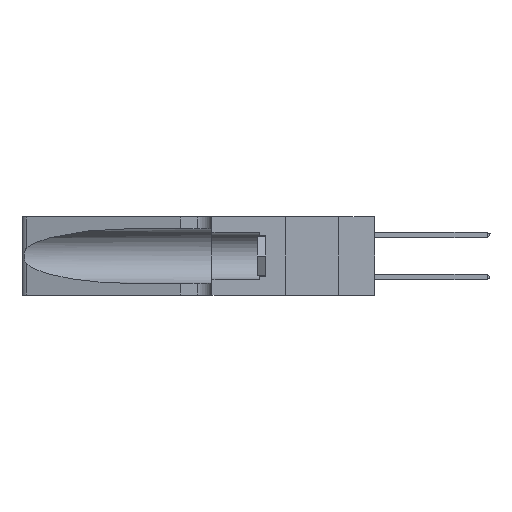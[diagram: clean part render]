
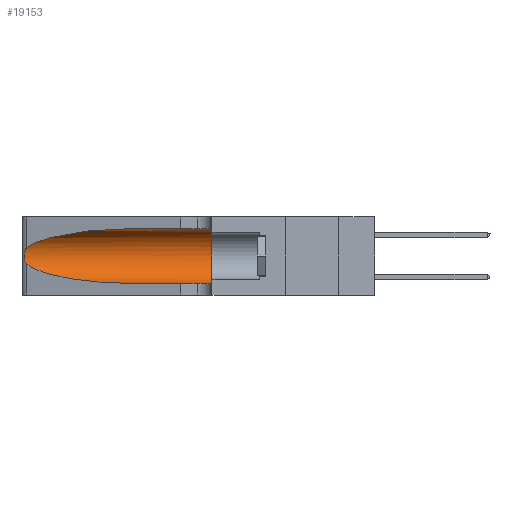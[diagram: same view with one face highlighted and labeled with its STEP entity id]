
A CAD part, left-side view. The second image highlights one B-rep face of the part: STEP entity #19153.
In plain terms, the highlighted cylindrical face has radius 3.308 mm (diameter 6.617 mm), a partial arc.
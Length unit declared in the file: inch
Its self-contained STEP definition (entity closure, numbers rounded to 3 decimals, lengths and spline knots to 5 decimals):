
#128 = EDGE_LOOP ( 'NONE', ( #16475, #12457, #3145, #19576, #9254, #17117 ) ) ;
#361 = CARTESIAN_POINT ( 'NONE',  ( 0.1305, 1.61858, 0.31525 ) ) ;
#1001 = CARTESIAN_POINT ( 'NONE',  ( 0.1305, 0.72297, 0.31525 ) ) ;
#1031 = DIRECTION ( 'NONE',  ( 0., -1., 0. ) ) ;
#1089 = CARTESIAN_POINT ( 'NONE',  ( 0.2373, 1.15595, 0.28018 ) ) ;
#1699 = AXIS2_PLACEMENT_3D ( 'NONE', #20190, #12353, #16362 ) ;
#2793 = VERTEX_POINT ( 'NONE', #5870 ) ;
#2833 = VERTEX_POINT ( 'NONE', #12127 ) ;
#3140 = EDGE_CURVE ( 'NONE', #2793, #24458, #7477, .T. ) ;
#3145 = ORIENTED_EDGE ( 'NONE', *, *, #16802, .T. ) ;
#3312 =( BOUNDED_CURVE ( )  B_SPLINE_CURVE ( 3, ( #18362, #6583, #24259, #16506 ),
 .UNSPECIFIED., .F., .F. ) 
 B_SPLINE_CURVE_WITH_KNOTS ( ( 4, 4 ),
 ( 3.44316, 4.71239 ),
 .UNSPECIFIED. ) 
 CURVE ( )  GEOMETRIC_REPRESENTATION_ITEM ( )  RATIONAL_B_SPLINE_CURVE ( ( 1., 0.87, 0.87, 1. ) ) 
 REPRESENTATION_ITEM ( '' )  );
#3843 = CARTESIAN_POINT ( 'NONE',  ( 0.25787, 1.23484, 0.2124 ) ) ;
#4177 = CARTESIAN_POINT ( 'NONE',  ( 0.25856, 1.23593, 0.16098 ) ) ;
#4266 = VERTEX_POINT ( 'NONE', #18389 ) ;
#4960 = CARTESIAN_POINT ( 'NONE',  ( 0.18966, 0.96281, 0.31525 ) ) ;
#5870 = CARTESIAN_POINT ( 'NONE',  ( 0.1305, 0.72297, 0.31525 ) ) ;
#6583 = CARTESIAN_POINT ( 'NONE',  ( 0.2373, 1.15595, 0.08982 ) ) ;
#6939 = CARTESIAN_POINT ( 'NONE',  ( 0.1305, 0.35, 0.05475 ) ) ;
#7477 =( BOUNDED_CURVE ( )  B_SPLINE_CURVE ( 3, ( #1001, #4960, #1089, #16830 ),
 .UNSPECIFIED., .F., .F. ) 
 B_SPLINE_CURVE_WITH_KNOTS ( ( 4, 4 ),
 ( 1.5708, 2.84003 ),
 .UNSPECIFIED. ) 
 CURVE ( )  GEOMETRIC_REPRESENTATION_ITEM ( )  RATIONAL_B_SPLINE_CURVE ( ( 1., 0.87, 0.87, 1. ) ) 
 REPRESENTATION_ITEM ( '' )  );
#7938 = CARTESIAN_POINT ( 'NONE',  ( 0.26017, 1.23833, 0.17102 ) ) ;
#8469 = CARTESIAN_POINT ( 'NONE',  ( 0.1305, 0.35, 0.185 ) ) ;
#8506 = VECTOR ( 'NONE', #16372, 39.37008 ) ;
#8920 = VERTEX_POINT ( 'NONE', #17496 ) ;
#9254 = ORIENTED_EDGE ( 'NONE', *, *, #16965, .F. ) ;
#9884 = EDGE_CURVE ( 'NONE', #24458, #4266, #23513, .T. ) ;
#10237 = CYLINDRICAL_SURFACE ( 'NONE', #1699, 0.13025 ) ;
#10624 = DIRECTION ( 'NONE',  ( 0., 0., 1. ) ) ;
#11306 = CARTESIAN_POINT ( 'NONE',  ( 0.25555, 1.22994, 0.2215 ) ) ;
#12127 = CARTESIAN_POINT ( 'NONE',  ( 0.1305, 0.72297, 0.05475 ) ) ;
#12353 = DIRECTION ( 'NONE',  ( 0., -1., 0. ) ) ;
#12457 = ORIENTED_EDGE ( 'NONE', *, *, #9884, .T. ) ;
#13435 = CARTESIAN_POINT ( 'NONE',  ( 0.25487, 1.22718, 0.22369 ) ) ;
#13534 = EDGE_CURVE ( 'NONE', #2833, #22809, #16464, .T. ) ;
#14095 = CARTESIAN_POINT ( 'NONE',  ( 0.25555, 1.22993, 0.14849 ) ) ;
#15099 = CIRCLE ( 'NONE', #20321, 0.13025 ) ;
#15268 = EDGE_CURVE ( 'NONE', #2793, #8920, #20416, .T. ) ;
#15723 = CARTESIAN_POINT ( 'NONE',  ( 0.26075, 1.23896, 0.178 ) ) ;
#16362 = DIRECTION ( 'NONE',  ( 0., 0., -1. ) ) ;
#16372 = DIRECTION ( 'NONE',  ( 0., -1., 0. ) ) ;
#16464 = LINE ( 'NONE', #20210, #8506 ) ;
#16475 = ORIENTED_EDGE ( 'NONE', *, *, #3140, .T. ) ;
#16506 = CARTESIAN_POINT ( 'NONE',  ( 0.1305, 0.72297, 0.05475 ) ) ;
#16802 = EDGE_CURVE ( 'NONE', #4266, #2833, #3312, .T. ) ;
#16830 = CARTESIAN_POINT ( 'NONE',  ( 0.25487, 1.22718, 0.22369 ) ) ;
#16965 = EDGE_CURVE ( 'NONE', #8920, #22809, #15099, .T. ) ;
#17117 = ORIENTED_EDGE ( 'NONE', *, *, #15268, .F. ) ;
#17466 = CARTESIAN_POINT ( 'NONE',  ( 0.25854, 1.2359, 0.20912 ) ) ;
#17496 = CARTESIAN_POINT ( 'NONE',  ( 0.1305, 0.35, 0.31525 ) ) ;
#17951 = VECTOR ( 'NONE', #1031, 39.37008 ) ;
#18276 = DIRECTION ( 'NONE',  ( 0., 1., 0. ) ) ;
#18362 = CARTESIAN_POINT ( 'NONE',  ( 0.25487, 1.22718, 0.14631 ) ) ;
#18389 = CARTESIAN_POINT ( 'NONE',  ( 0.25487, 1.22718, 0.14631 ) ) ;
#19036 = CARTESIAN_POINT ( 'NONE',  ( 0.25639, 1.23184, 0.21858 ) ) ;
#19153 = ADVANCED_FACE ( 'NONE', ( #21595 ), #10237, .F. ) ;
#19576 = ORIENTED_EDGE ( 'NONE', *, *, #13534, .T. ) ;
#19637 = CARTESIAN_POINT ( 'NONE',  ( 0.26075, 1.23896, 0.19203 ) ) ;
#19891 = CARTESIAN_POINT ( 'NONE',  ( 0.25789, 1.23486, 0.15765 ) ) ;
#20190 = CARTESIAN_POINT ( 'NONE',  ( 0.1305, 1.61858, 0.185 ) ) ;
#20210 = CARTESIAN_POINT ( 'NONE',  ( 0.1305, 1.61858, 0.05475 ) ) ;
#20321 = AXIS2_PLACEMENT_3D ( 'NONE', #8469, #18276, #10624 ) ;
#20416 = LINE ( 'NONE', #361, #17951 ) ;
#21422 = CARTESIAN_POINT ( 'NONE',  ( 0.26018, 1.23835, 0.19895 ) ) ;
#21595 = FACE_OUTER_BOUND ( 'NONE', #128, .T. ) ;
#22081 = CARTESIAN_POINT ( 'NONE',  ( 0.25487, 1.22718, 0.14631 ) ) ;
#22809 = VERTEX_POINT ( 'NONE', #6939 ) ;
#23513 = B_SPLINE_CURVE_WITH_KNOTS ( 'NONE', 3,
 ( #13435, #11306, #19036, #3843, #17466, #21422, #19637, #15723, #7938, #4177, #19891, #23802, #14095, #22081 ),
 .UNSPECIFIED., .F., .F.,
 ( 4, 2, 2, 2, 2, 2, 4 ),
 ( 0., 0.00027, 0.00053, 0.00107, 0.0016, 0.00187, 0.00214 ),
 .UNSPECIFIED. ) ;
#23802 = CARTESIAN_POINT ( 'NONE',  ( 0.25639, 1.23186, 0.15144 ) ) ;
#24259 = CARTESIAN_POINT ( 'NONE',  ( 0.18966, 0.96281, 0.05475 ) ) ;
#24458 = VERTEX_POINT ( 'NONE', #24982 ) ;
#24982 = CARTESIAN_POINT ( 'NONE',  ( 0.25487, 1.22718, 0.22369 ) ) ;
